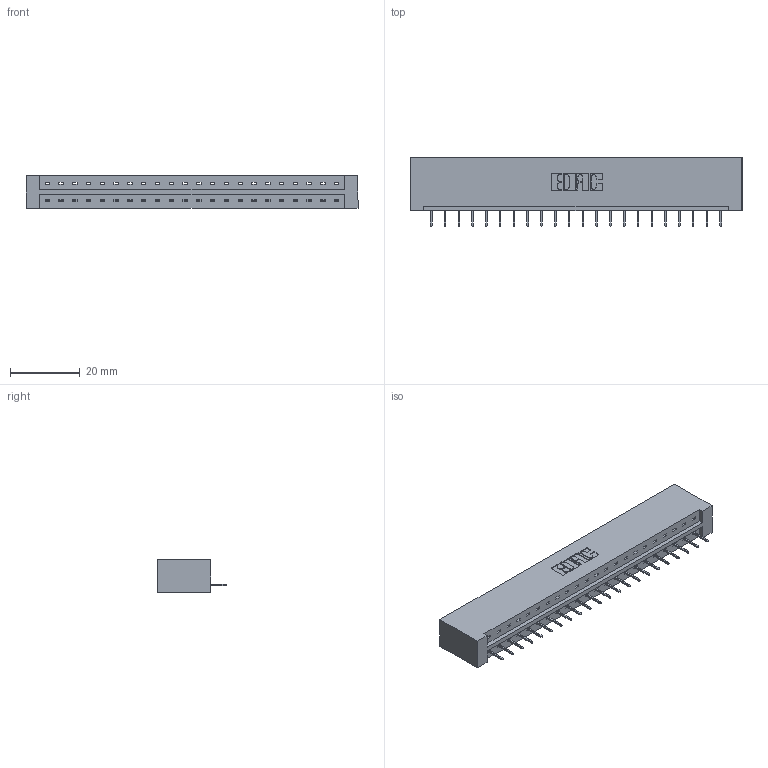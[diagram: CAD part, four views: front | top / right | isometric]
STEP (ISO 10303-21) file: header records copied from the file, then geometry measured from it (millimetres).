
FILE_DESCRIPTION (( 'STEP AP203' ), '1' );
FILE_NAME ('333-022-524-101.STEP', '2018-08-02T01:57:51', ( '' ), ( '' ), 'SwSTEP 2.0', 'SolidWorks 2016', '' );
FILE_SCHEMA (( 'CONFIG_CONTROL_DESIGN' ));
Length unit declared in the file: inch
Products named in the file (3): 333 Part_Lugless; 345-292-001_345-293-124; 333-022-524-101
Assembly tree (23 placements, depth 2):
  333-022-524-101
    333 Part_Lugless
    345-292-001_345-293-124  x22
Bounding box: 95.43 x 19.69 x 9.4 mm (x, y, z)
Volume: 9956.6 mm3; surface area: 10299.8 mm2
Topology: 23 solids, 23 shells, 1470 faces, 4247 edges, 2742 vertices
Faces by surface type: plane 1122, cylinder 348
Entity records: 15833 total; most frequent: CARTESIAN_POINT 2740, ORIENTED_EDGE 2698, DIRECTION 2345, EDGE_CURVE 1349, VECTOR 1233, LINE 1233, VERTEX_POINT 894, AXIS2_PLACEMENT_3D 556
